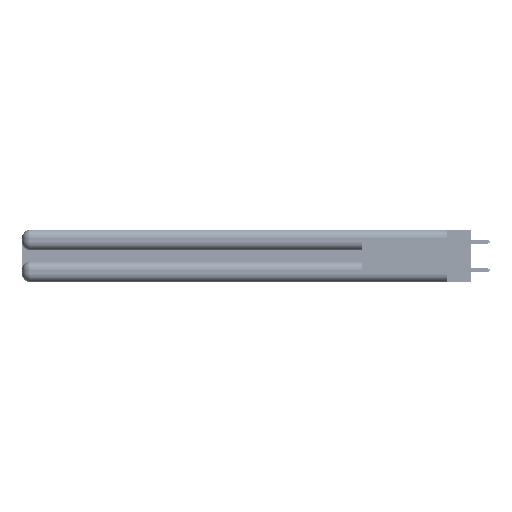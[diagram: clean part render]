
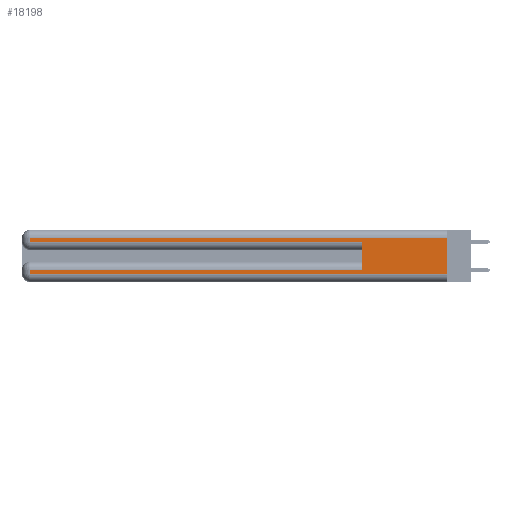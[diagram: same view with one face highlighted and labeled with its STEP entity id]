
A CAD part, left-side view. The second image highlights one B-rep face of the part: STEP entity #18198.
In plain terms, the highlighted planar face has unit normal (-1, 0, 0).
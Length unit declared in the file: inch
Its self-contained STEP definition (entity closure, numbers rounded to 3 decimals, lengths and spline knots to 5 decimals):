
#1711 = DIRECTION ( 'NONE',  ( 0., 0., -1. ) ) ;
#3488 = VECTOR ( 'NONE', #51232, 39.37008 ) ;
#4034 = CARTESIAN_POINT ( 'NONE',  ( 0., 0., 0.085 ) ) ;
#4359 = CARTESIAN_POINT ( 'NONE',  ( 0., 2.94, 0.06 ) ) ;
#4730 = VERTEX_POINT ( 'NONE', #37695 ) ;
#5173 = DIRECTION ( 'NONE',  ( 0., 0., -1. ) ) ;
#7820 = EDGE_CURVE ( 'NONE', #9152, #47737, #15346, .T. ) ;
#7896 = DIRECTION ( 'NONE',  ( 0., 0., 1. ) ) ;
#7984 = LINE ( 'NONE', #35746, #19956 ) ;
#8691 = LINE ( 'NONE', #28712, #43015 ) ;
#9152 = VERTEX_POINT ( 'NONE', #28885 ) ;
#9771 = AXIS2_PLACEMENT_3D ( 'NONE', #33179, #24335, #55368 ) ;
#9984 = CARTESIAN_POINT ( 'NONE',  ( 0., 2.94, 0.085 ) ) ;
#12074 = ORIENTED_EDGE ( 'NONE', *, *, #27756, .T. ) ;
#13237 = EDGE_CURVE ( 'NONE', #42514, #57321, #8691, .T. ) ;
#14878 = DIRECTION ( 'NONE',  ( 0., 1., 0. ) ) ;
#15311 = PLANE ( 'NONE',  #9771 ) ;
#15346 = LINE ( 'NONE', #49880, #25883 ) ;
#15625 = CARTESIAN_POINT ( 'NONE',  ( 0., 0., 0.285 ) ) ;
#15777 = EDGE_CURVE ( 'NONE', #17879, #9152, #43387, .T. ) ;
#17475 = VECTOR ( 'NONE', #54781, 39.37008 ) ;
#17730 = ORIENTED_EDGE ( 'NONE', *, *, #56580, .T. ) ;
#17879 = VERTEX_POINT ( 'NONE', #26740 ) ;
#18198 = ADVANCED_FACE ( 'NONE', ( #45301 ), #15311, .F. ) ;
#18964 = EDGE_LOOP ( 'NONE', ( #42214, #19812, #55273, #12074, #24054, #17730, #41542, #54610 ) ) ;
#19802 = EDGE_CURVE ( 'NONE', #4730, #22829, #47186, .T. ) ;
#19812 = ORIENTED_EDGE ( 'NONE', *, *, #15777, .T. ) ;
#19956 = VECTOR ( 'NONE', #44609, 39.37008 ) ;
#20659 = CARTESIAN_POINT ( 'NONE',  ( 0., 0.6, 0.285 ) ) ;
#22829 = VERTEX_POINT ( 'NONE', #20659 ) ;
#24054 = ORIENTED_EDGE ( 'NONE', *, *, #19802, .F. ) ;
#24335 = DIRECTION ( 'NONE',  ( 1., 0., 0. ) ) ;
#24963 = EDGE_CURVE ( 'NONE', #17879, #56195, #7984, .T. ) ;
#25883 = VECTOR ( 'NONE', #5173, 39.37008 ) ;
#26740 = CARTESIAN_POINT ( 'NONE',  ( 0., 0., 0.31 ) ) ;
#27756 = EDGE_CURVE ( 'NONE', #47737, #22829, #46907, .T. ) ;
#28712 = CARTESIAN_POINT ( 'NONE',  ( 0., 2.94, 0.37 ) ) ;
#28885 = CARTESIAN_POINT ( 'NONE',  ( 0., 2.94, 0.31 ) ) ;
#31472 = EDGE_CURVE ( 'NONE', #57321, #56195, #41281, .T. ) ;
#31515 = VECTOR ( 'NONE', #35525, 39.37008 ) ;
#31616 = VECTOR ( 'NONE', #14878, 39.37008 ) ;
#32437 = CARTESIAN_POINT ( 'NONE',  ( 0., 0., 0.06 ) ) ;
#32669 = VECTOR ( 'NONE', #7896, 39.37008 ) ;
#32764 = CARTESIAN_POINT ( 'NONE',  ( 0., 0., 0.31 ) ) ;
#32777 = CARTESIAN_POINT ( 'NONE',  ( 0., 0., 0.06 ) ) ;
#33179 = CARTESIAN_POINT ( 'NONE',  ( 0., 0., 0.37 ) ) ;
#35525 = DIRECTION ( 'NONE',  ( 0., 1., 0. ) ) ;
#35746 = CARTESIAN_POINT ( 'NONE',  ( 0., 0., 0.37 ) ) ;
#37695 = CARTESIAN_POINT ( 'NONE',  ( 0., 0.6, 0.085 ) ) ;
#41281 = LINE ( 'NONE', #32777, #17475 ) ;
#41542 = ORIENTED_EDGE ( 'NONE', *, *, #13237, .T. ) ;
#42214 = ORIENTED_EDGE ( 'NONE', *, *, #24963, .F. ) ;
#42514 = VERTEX_POINT ( 'NONE', #9984 ) ;
#43015 = VECTOR ( 'NONE', #1711, 39.37008 ) ;
#43387 = LINE ( 'NONE', #32764, #31616 ) ;
#43509 = CARTESIAN_POINT ( 'NONE',  ( 0., 0.6, 0.145 ) ) ;
#44609 = DIRECTION ( 'NONE',  ( 0., 0., -1. ) ) ;
#45301 = FACE_OUTER_BOUND ( 'NONE', #18964, .T. ) ;
#46907 = LINE ( 'NONE', #15625, #3488 ) ;
#47186 = LINE ( 'NONE', #43509, #32669 ) ;
#47737 = VERTEX_POINT ( 'NONE', #55848 ) ;
#49880 = CARTESIAN_POINT ( 'NONE',  ( 0., 2.94, 0.37 ) ) ;
#51232 = DIRECTION ( 'NONE',  ( 0., -1., 0. ) ) ;
#53619 = LINE ( 'NONE', #4034, #31515 ) ;
#54610 = ORIENTED_EDGE ( 'NONE', *, *, #31472, .T. ) ;
#54781 = DIRECTION ( 'NONE',  ( 0., -1., 0. ) ) ;
#55273 = ORIENTED_EDGE ( 'NONE', *, *, #7820, .T. ) ;
#55368 = DIRECTION ( 'NONE',  ( 0., 0., -1. ) ) ;
#55848 = CARTESIAN_POINT ( 'NONE',  ( 0., 2.94, 0.285 ) ) ;
#56195 = VERTEX_POINT ( 'NONE', #32437 ) ;
#56580 = EDGE_CURVE ( 'NONE', #4730, #42514, #53619, .T. ) ;
#57321 = VERTEX_POINT ( 'NONE', #4359 ) ;
